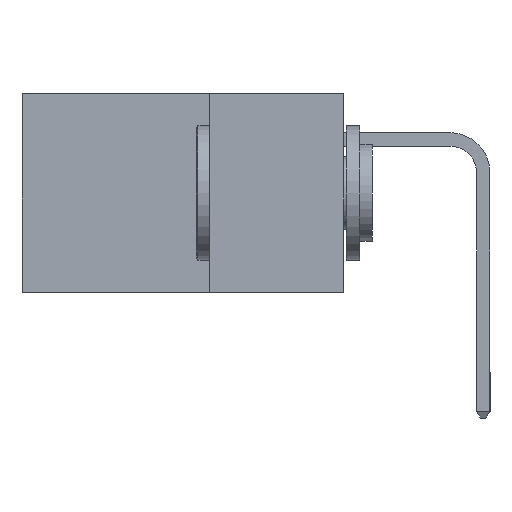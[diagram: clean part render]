
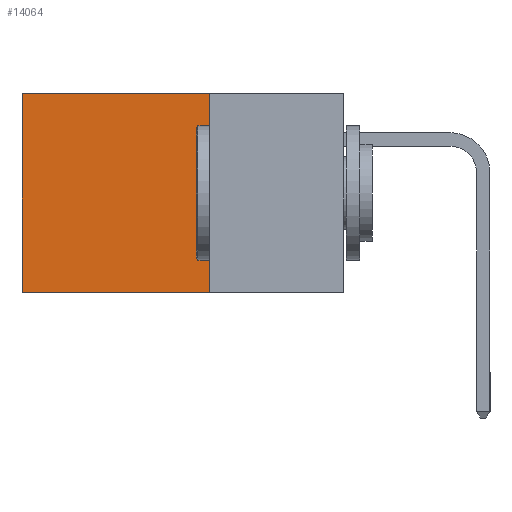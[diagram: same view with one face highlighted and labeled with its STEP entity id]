
A CAD part, left-side view. The second image highlights one B-rep face of the part: STEP entity #14064.
In plain terms, the highlighted planar face has unit normal (-1, 0, 0).
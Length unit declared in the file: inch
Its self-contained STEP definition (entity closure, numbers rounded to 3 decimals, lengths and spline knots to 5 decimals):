
#1300 = EDGE_CURVE ( 'NONE', #9979, #5294, #2183, .T. ) ;
#1504 = CARTESIAN_POINT ( 'NONE',  ( 0.298, 0.6, 0. ) ) ;
#1622 = ORIENTED_EDGE ( 'NONE', *, *, #13838, .F. ) ;
#2183 = LINE ( 'NONE', #4597, #10193 ) ;
#2334 = VECTOR ( 'NONE', #13234, 39.37008 ) ;
#2365 = CARTESIAN_POINT ( 'NONE',  ( 0.298, 0.6, -0.37 ) ) ;
#2410 = VERTEX_POINT ( 'NONE', #8550 ) ;
#3309 = LINE ( 'NONE', #5105, #12859 ) ;
#3619 = ORIENTED_EDGE ( 'NONE', *, *, #1300, .T. ) ;
#3690 = PLANE ( 'NONE',  #6422 ) ;
#3692 = LINE ( 'NONE', #1504, #5226 ) ;
#4597 = CARTESIAN_POINT ( 'NONE',  ( 0.298, 0.25, 0. ) ) ;
#4791 = DIRECTION ( 'NONE',  ( 0., 0., -1. ) ) ;
#4924 = DIRECTION ( 'NONE',  ( 1., 0., 0. ) ) ;
#5105 = CARTESIAN_POINT ( 'NONE',  ( 0.298, 0.25, 0. ) ) ;
#5226 = VECTOR ( 'NONE', #5923, 39.37008 ) ;
#5294 = VERTEX_POINT ( 'NONE', #7801 ) ;
#5593 = CARTESIAN_POINT ( 'NONE',  ( 0.298, 0.25, -0.37 ) ) ;
#5923 = DIRECTION ( 'NONE',  ( 0., 0., -1. ) ) ;
#6190 = DIRECTION ( 'NONE',  ( 0., 0., -1. ) ) ;
#6226 = CARTESIAN_POINT ( 'NONE',  ( 0.298, 0.25, 0. ) ) ;
#6422 = AXIS2_PLACEMENT_3D ( 'NONE', #11302, #4924, #4791 ) ;
#6906 = EDGE_LOOP ( 'NONE', ( #11951, #1622, #10689, #3619 ) ) ;
#7801 = CARTESIAN_POINT ( 'NONE',  ( 0.298, 0.6, 0. ) ) ;
#8156 = EDGE_CURVE ( 'NONE', #9979, #2410, #3309, .T. ) ;
#8550 = CARTESIAN_POINT ( 'NONE',  ( 0.298, 0.25, -0.37 ) ) ;
#9017 = VERTEX_POINT ( 'NONE', #2365 ) ;
#9319 = LINE ( 'NONE', #5593, #2334 ) ;
#9979 = VERTEX_POINT ( 'NONE', #6226 ) ;
#10154 = DIRECTION ( 'NONE',  ( 0., 1., 0. ) ) ;
#10193 = VECTOR ( 'NONE', #10154, 39.37008 ) ;
#10689 = ORIENTED_EDGE ( 'NONE', *, *, #8156, .F. ) ;
#11302 = CARTESIAN_POINT ( 'NONE',  ( 0.298, 0.25, 0. ) ) ;
#11951 = ORIENTED_EDGE ( 'NONE', *, *, #14022, .T. ) ;
#12050 = FACE_OUTER_BOUND ( 'NONE', #6906, .T. ) ;
#12859 = VECTOR ( 'NONE', #6190, 39.37008 ) ;
#13234 = DIRECTION ( 'NONE',  ( 0., 1., 0. ) ) ;
#13838 = EDGE_CURVE ( 'NONE', #2410, #9017, #9319, .T. ) ;
#14022 = EDGE_CURVE ( 'NONE', #5294, #9017, #3692, .T. ) ;
#14064 = ADVANCED_FACE ( 'NONE', ( #12050 ), #3690, .F. ) ;
